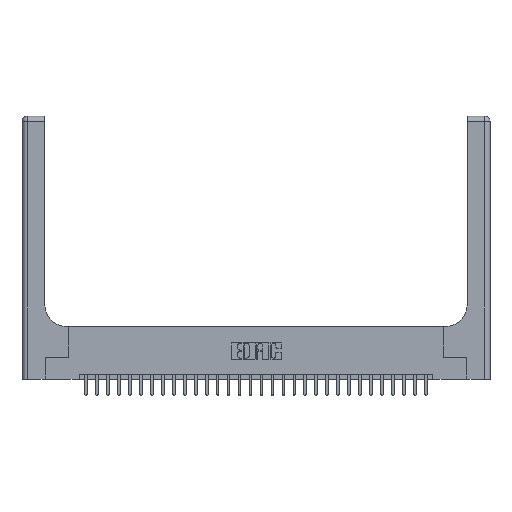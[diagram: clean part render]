
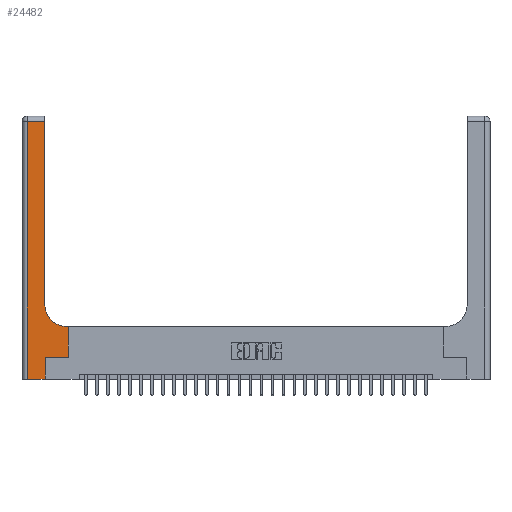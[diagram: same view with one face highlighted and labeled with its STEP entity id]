
A CAD part, top view. The second image highlights one B-rep face of the part: STEP entity #24482.
In plain terms, the highlighted planar face has unit normal (0, 0, 1).
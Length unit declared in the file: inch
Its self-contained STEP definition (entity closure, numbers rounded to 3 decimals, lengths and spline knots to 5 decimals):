
#98 = CARTESIAN_POINT ( 'NONE',  ( 0., 3., 0.37 ) ) ;
#226 = DIRECTION ( 'NONE',  ( -1., 0., 0. ) ) ;
#544 = VECTOR ( 'NONE', #26383, 39.37008 ) ;
#975 = CARTESIAN_POINT ( 'NONE',  ( 0.265, 0.25, 0.37 ) ) ;
#1498 = VERTEX_POINT ( 'NONE', #19908 ) ;
#1832 = LINE ( 'NONE', #2517, #14567 ) ;
#2233 = CARTESIAN_POINT ( 'NONE',  ( 0.265, 0., 0.37 ) ) ;
#2253 = VERTEX_POINT ( 'NONE', #6496 ) ;
#2361 = VECTOR ( 'NONE', #15690, 39.37008 ) ;
#2517 = CARTESIAN_POINT ( 'NONE',  ( 0., 0., 0.37 ) ) ;
#4332 = AXIS2_PLACEMENT_3D ( 'NONE', #5485, #12002, #5460 ) ;
#4428 = VERTEX_POINT ( 'NONE', #8825 ) ;
#4772 = LINE ( 'NONE', #17944, #2361 ) ;
#4899 = DIRECTION ( 'NONE',  ( 0., 0., -1. ) ) ;
#5460 = DIRECTION ( 'NONE',  ( 1., 0., 0. ) ) ;
#5485 = CARTESIAN_POINT ( 'NONE',  ( 0.51, 0.85, 0.37 ) ) ;
#5620 = EDGE_CURVE ( 'NONE', #20094, #11594, #18818, .T. ) ;
#5894 = EDGE_CURVE ( 'NONE', #1498, #15967, #6440, .T. ) ;
#6299 = CARTESIAN_POINT ( 'NONE',  ( 0., 2.94, 0.37 ) ) ;
#6440 = LINE ( 'NONE', #6299, #26987 ) ;
#6496 = CARTESIAN_POINT ( 'NONE',  ( 0.528, 0.25, 0.37 ) ) ;
#6737 = VERTEX_POINT ( 'NONE', #7493 ) ;
#6862 = LINE ( 'NONE', #15640, #9282 ) ;
#7025 = FACE_OUTER_BOUND ( 'NONE', #21529, .T. ) ;
#7422 = EDGE_CURVE ( 'NONE', #11594, #1498, #6862, .T. ) ;
#7493 = CARTESIAN_POINT ( 'NONE',  ( 0.265, 0., 0.37 ) ) ;
#8472 = LINE ( 'NONE', #2233, #17769 ) ;
#8794 = CARTESIAN_POINT ( 'NONE',  ( 0.06, 0., 0.37 ) ) ;
#8825 = CARTESIAN_POINT ( 'NONE',  ( 0.528, 0.6, 0.37 ) ) ;
#9113 = LINE ( 'NONE', #17750, #544 ) ;
#9282 = VECTOR ( 'NONE', #15217, 39.37008 ) ;
#9311 = AXIS2_PLACEMENT_3D ( 'NONE', #98, #4899, #226 ) ;
#10299 = EDGE_CURVE ( 'NONE', #2253, #4428, #9113, .T. ) ;
#10738 = ORIENTED_EDGE ( 'NONE', *, *, #22704, .T. ) ;
#10879 = ORIENTED_EDGE ( 'NONE', *, *, #10299, .T. ) ;
#11204 = VERTEX_POINT ( 'NONE', #975 ) ;
#11594 = VERTEX_POINT ( 'NONE', #15256 ) ;
#12002 = DIRECTION ( 'NONE',  ( 0., 0., -1. ) ) ;
#12745 = EDGE_CURVE ( 'NONE', #6737, #11204, #8472, .T. ) ;
#13061 = CARTESIAN_POINT ( 'NONE',  ( 0.06, 2.94, 0.37 ) ) ;
#13144 = CARTESIAN_POINT ( 'NONE',  ( 0.265, 0.25, 0.37 ) ) ;
#14562 = DIRECTION ( 'NONE',  ( 0., 1., 0. ) ) ;
#14567 = VECTOR ( 'NONE', #22215, 39.37008 ) ;
#14930 = DIRECTION ( 'NONE',  ( -1., 0., 0. ) ) ;
#15217 = DIRECTION ( 'NONE',  ( 0., 1., 0. ) ) ;
#15230 = CARTESIAN_POINT ( 'NONE',  ( 0.51, 0.6, 0.37 ) ) ;
#15256 = CARTESIAN_POINT ( 'NONE',  ( 0.26, 0.85, 0.37 ) ) ;
#15269 = DIRECTION ( 'NONE',  ( 1., 0., 0. ) ) ;
#15466 = VECTOR ( 'NONE', #15269, 39.37008 ) ;
#15640 = CARTESIAN_POINT ( 'NONE',  ( 0.26, 3., 0.37 ) ) ;
#15690 = DIRECTION ( 'NONE',  ( -1., 0., 0. ) ) ;
#15967 = VERTEX_POINT ( 'NONE', #13061 ) ;
#16378 = ORIENTED_EDGE ( 'NONE', *, *, #5620, .T. ) ;
#17020 = DIRECTION ( 'NONE',  ( 0., -1., 0. ) ) ;
#17655 = PLANE ( 'NONE',  #9311 ) ;
#17750 = CARTESIAN_POINT ( 'NONE',  ( 0.528, 0.25, 0.37 ) ) ;
#17769 = VECTOR ( 'NONE', #14562, 39.37008 ) ;
#17944 = CARTESIAN_POINT ( 'NONE',  ( 0.26, 0.6, 0.37 ) ) ;
#18074 = ORIENTED_EDGE ( 'NONE', *, *, #25059, .T. ) ;
#18127 = EDGE_CURVE ( 'NONE', #4428, #20094, #4772, .T. ) ;
#18171 = EDGE_CURVE ( 'NONE', #11204, #2253, #21919, .T. ) ;
#18284 = ORIENTED_EDGE ( 'NONE', *, *, #18127, .T. ) ;
#18818 = CIRCLE ( 'NONE', #4332, 0.25 ) ;
#19908 = CARTESIAN_POINT ( 'NONE',  ( 0.26, 2.94, 0.37 ) ) ;
#20094 = VERTEX_POINT ( 'NONE', #15230 ) ;
#21089 = VECTOR ( 'NONE', #17020, 39.37008 ) ;
#21471 = ORIENTED_EDGE ( 'NONE', *, *, #5894, .T. ) ;
#21529 = EDGE_LOOP ( 'NONE', ( #23371, #21471, #18074, #10738, #27172, #23936, #10879, #18284, #16378 ) ) ;
#21919 = LINE ( 'NONE', #13144, #15466 ) ;
#22215 = DIRECTION ( 'NONE',  ( 1., 0., 0. ) ) ;
#22704 = EDGE_CURVE ( 'NONE', #24065, #6737, #1832, .T. ) ;
#22980 = CARTESIAN_POINT ( 'NONE',  ( 0.06, 3., 0.37 ) ) ;
#23114 = LINE ( 'NONE', #22980, #21089 ) ;
#23371 = ORIENTED_EDGE ( 'NONE', *, *, #7422, .T. ) ;
#23936 = ORIENTED_EDGE ( 'NONE', *, *, #18171, .T. ) ;
#24065 = VERTEX_POINT ( 'NONE', #8794 ) ;
#24482 = ADVANCED_FACE ( 'NONE', ( #7025 ), #17655, .F. ) ;
#25059 = EDGE_CURVE ( 'NONE', #15967, #24065, #23114, .T. ) ;
#26383 = DIRECTION ( 'NONE',  ( 0., 1., 0. ) ) ;
#26987 = VECTOR ( 'NONE', #14930, 39.37008 ) ;
#27172 = ORIENTED_EDGE ( 'NONE', *, *, #12745, .T. ) ;
